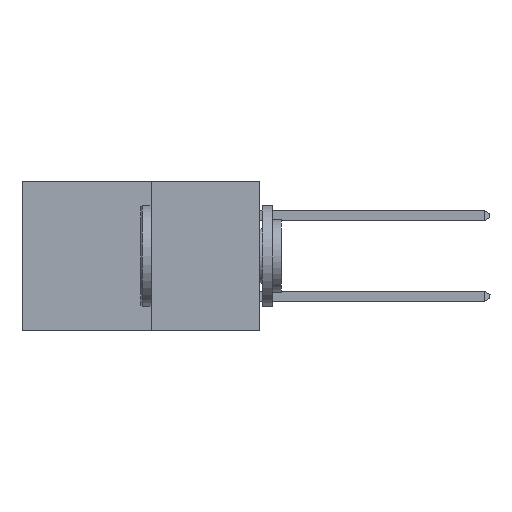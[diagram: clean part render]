
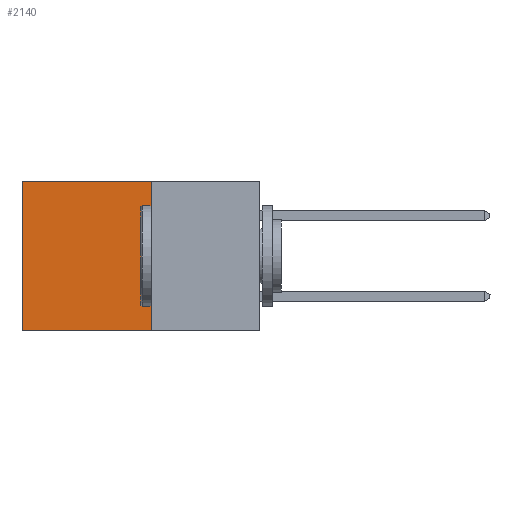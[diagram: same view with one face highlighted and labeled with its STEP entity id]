
A CAD part, left-side view. The second image highlights one B-rep face of the part: STEP entity #2140.
In plain terms, the highlighted planar face has unit normal (-1, 0, 0).
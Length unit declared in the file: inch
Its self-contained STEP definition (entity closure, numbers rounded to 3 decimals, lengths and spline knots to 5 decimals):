
#289 = CARTESIAN_POINT ( 'NONE',  ( 0.277, 0.59, -0.37 ) ) ;
#509 = FACE_OUTER_BOUND ( 'NONE', #6662, .T. ) ;
#1442 = VECTOR ( 'NONE', #2066, 39.37008 ) ;
#1900 = EDGE_CURVE ( 'NONE', #4865, #4286, #5624, .T. ) ;
#2066 = DIRECTION ( 'NONE',  ( 0., 0., -1. ) ) ;
#2140 = ADVANCED_FACE ( 'NONE', ( #509 ), #5802, .F. ) ;
#2437 = EDGE_CURVE ( 'NONE', #7829, #4865, #3800, .T. ) ;
#2570 = VECTOR ( 'NONE', #3287, 39.37008 ) ;
#2956 = LINE ( 'NONE', #9429, #6962 ) ;
#3287 = DIRECTION ( 'NONE',  ( 0., 1., 0. ) ) ;
#3800 = LINE ( 'NONE', #3997, #1442 ) ;
#3987 = VERTEX_POINT ( 'NONE', #8372 ) ;
#3997 = CARTESIAN_POINT ( 'NONE',  ( 0.277, 0.27, -0.37 ) ) ;
#4286 = VERTEX_POINT ( 'NONE', #289 ) ;
#4865 = VERTEX_POINT ( 'NONE', #8350 ) ;
#5209 = DIRECTION ( 'NONE',  ( 0., 0., -1. ) ) ;
#5259 = DIRECTION ( 'NONE',  ( 1., 0., 0. ) ) ;
#5336 = EDGE_CURVE ( 'NONE', #7829, #3987, #6854, .T. ) ;
#5343 = AXIS2_PLACEMENT_3D ( 'NONE', #8117, #5259, #5209 ) ;
#5471 = EDGE_CURVE ( 'NONE', #3987, #4286, #2956, .T. ) ;
#5624 = LINE ( 'NONE', #6733, #9333 ) ;
#5802 = PLANE ( 'NONE',  #5343 ) ;
#5872 = ORIENTED_EDGE ( 'NONE', *, *, #5471, .T. ) ;
#5957 = ORIENTED_EDGE ( 'NONE', *, *, #1900, .F. ) ;
#6010 = DIRECTION ( 'NONE',  ( 0., 1., 0. ) ) ;
#6012 = ORIENTED_EDGE ( 'NONE', *, *, #2437, .F. ) ;
#6032 = DIRECTION ( 'NONE',  ( 0., 0., -1. ) ) ;
#6115 = ORIENTED_EDGE ( 'NONE', *, *, #5336, .T. ) ;
#6159 = CARTESIAN_POINT ( 'NONE',  ( 0.277, 0.27, 0. ) ) ;
#6662 = EDGE_LOOP ( 'NONE', ( #5872, #5957, #6012, #6115 ) ) ;
#6733 = CARTESIAN_POINT ( 'NONE',  ( 0.277, 0.27, -0.37 ) ) ;
#6854 = LINE ( 'NONE', #7866, #2570 ) ;
#6962 = VECTOR ( 'NONE', #6032, 39.37008 ) ;
#7829 = VERTEX_POINT ( 'NONE', #6159 ) ;
#7866 = CARTESIAN_POINT ( 'NONE',  ( 0.277, 0.27, 0. ) ) ;
#8117 = CARTESIAN_POINT ( 'NONE',  ( 0.277, 0.27, -0.37 ) ) ;
#8350 = CARTESIAN_POINT ( 'NONE',  ( 0.277, 0.27, -0.37 ) ) ;
#8372 = CARTESIAN_POINT ( 'NONE',  ( 0.277, 0.59, 0. ) ) ;
#9333 = VECTOR ( 'NONE', #6010, 39.37008 ) ;
#9429 = CARTESIAN_POINT ( 'NONE',  ( 0.277, 0.59, -0.37 ) ) ;
